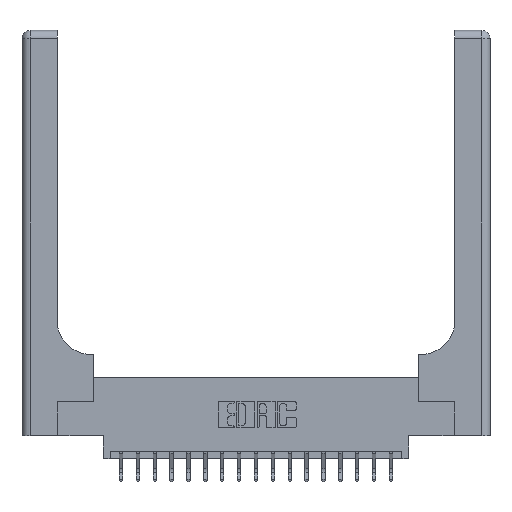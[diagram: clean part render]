
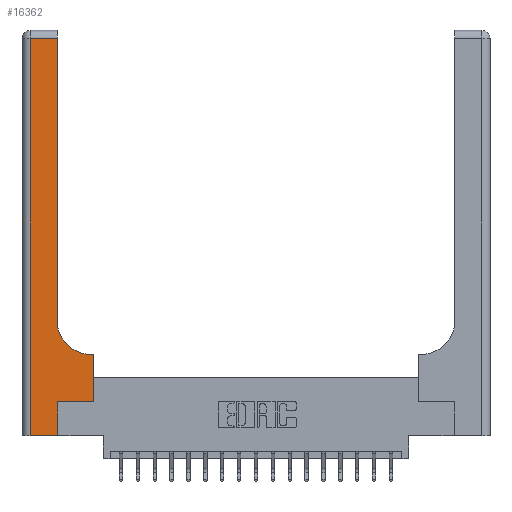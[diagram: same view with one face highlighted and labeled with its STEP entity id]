
A CAD part, top view. The second image highlights one B-rep face of the part: STEP entity #16362.
In plain terms, the highlighted planar face has unit normal (0, 0, 1).
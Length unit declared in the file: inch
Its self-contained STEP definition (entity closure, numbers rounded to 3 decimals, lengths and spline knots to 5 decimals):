
#475 = CARTESIAN_POINT ( 'NONE',  ( 0., 0., 0.37 ) ) ;
#522 = ORIENTED_EDGE ( 'NONE', *, *, #2065, .T. ) ;
#551 = DIRECTION ( 'NONE',  ( -1., 0., 0. ) ) ;
#961 = VERTEX_POINT ( 'NONE', #5490 ) ;
#1096 = DIRECTION ( 'NONE',  ( 0., 1., 0. ) ) ;
#1474 = DIRECTION ( 'NONE',  ( 0., 1., 0. ) ) ;
#1611 = VERTEX_POINT ( 'NONE', #2982 ) ;
#1693 = VECTOR ( 'NONE', #17607, 39.37008 ) ;
#1705 = VECTOR ( 'NONE', #16357, 39.37008 ) ;
#2053 = ORIENTED_EDGE ( 'NONE', *, *, #19436, .T. ) ;
#2065 = EDGE_CURVE ( 'NONE', #6285, #18009, #5100, .T. ) ;
#2177 = CARTESIAN_POINT ( 'NONE',  ( 0., 2.94, 0.37 ) ) ;
#2196 = CARTESIAN_POINT ( 'NONE',  ( 0.26, 0.6, 0.37 ) ) ;
#2361 = ORIENTED_EDGE ( 'NONE', *, *, #8511, .T. ) ;
#2476 = EDGE_CURVE ( 'NONE', #10745, #961, #14291, .T. ) ;
#2827 = CIRCLE ( 'NONE', #11440, 0.25 ) ;
#2853 = LINE ( 'NONE', #15486, #19802 ) ;
#2982 = CARTESIAN_POINT ( 'NONE',  ( 0.265, 0.25, 0.37 ) ) ;
#3101 = EDGE_CURVE ( 'NONE', #16613, #10745, #2853, .T. ) ;
#3130 = VERTEX_POINT ( 'NONE', #15181 ) ;
#3337 = CARTESIAN_POINT ( 'NONE',  ( 0.26, 0.85, 0.37 ) ) ;
#3581 = CARTESIAN_POINT ( 'NONE',  ( 0.26, 2.94, 0.37 ) ) ;
#4797 = CARTESIAN_POINT ( 'NONE',  ( 0.528, 0.6, 0.37 ) ) ;
#4808 = DIRECTION ( 'NONE',  ( 1., 0., 0. ) ) ;
#5100 = LINE ( 'NONE', #2196, #17167 ) ;
#5184 = VECTOR ( 'NONE', #4808, 39.37008 ) ;
#5490 = CARTESIAN_POINT ( 'NONE',  ( 0.06, 2.94, 0.37 ) ) ;
#5748 = EDGE_CURVE ( 'NONE', #961, #12472, #14971, .T. ) ;
#6152 = LINE ( 'NONE', #10940, #5184 ) ;
#6179 = DIRECTION ( 'NONE',  ( 0., 0., -1. ) ) ;
#6285 = VERTEX_POINT ( 'NONE', #4797 ) ;
#7074 = VERTEX_POINT ( 'NONE', #17645 ) ;
#8040 = DIRECTION ( 'NONE',  ( 1., 0., 0. ) ) ;
#8334 = FACE_OUTER_BOUND ( 'NONE', #10385, .T. ) ;
#8359 = CARTESIAN_POINT ( 'NONE',  ( 0.06, 3., 0.37 ) ) ;
#8511 = EDGE_CURVE ( 'NONE', #3130, #6285, #14005, .T. ) ;
#8544 = ORIENTED_EDGE ( 'NONE', *, *, #9188, .T. ) ;
#8663 = DIRECTION ( 'NONE',  ( 0., 0., -1. ) ) ;
#9188 = EDGE_CURVE ( 'NONE', #12472, #7074, #13227, .T. ) ;
#9408 = VECTOR ( 'NONE', #1474, 39.37008 ) ;
#10385 = EDGE_LOOP ( 'NONE', ( #17080, #19783, #10804, #8544, #2053, #17909, #2361, #522, #10898 ) ) ;
#10534 = EDGE_CURVE ( 'NONE', #18009, #16613, #2827, .T. ) ;
#10745 = VERTEX_POINT ( 'NONE', #3581 ) ;
#10804 = ORIENTED_EDGE ( 'NONE', *, *, #5748, .T. ) ;
#10898 = ORIENTED_EDGE ( 'NONE', *, *, #10534, .T. ) ;
#10940 = CARTESIAN_POINT ( 'NONE',  ( 0.265, 0.25, 0.37 ) ) ;
#11214 = LINE ( 'NONE', #14488, #1693 ) ;
#11440 = AXIS2_PLACEMENT_3D ( 'NONE', #15609, #6179, #8040 ) ;
#12072 = VECTOR ( 'NONE', #19526, 39.37008 ) ;
#12472 = VERTEX_POINT ( 'NONE', #16397 ) ;
#12721 = EDGE_CURVE ( 'NONE', #1611, #3130, #6152, .T. ) ;
#13227 = LINE ( 'NONE', #475, #12072 ) ;
#13960 = VECTOR ( 'NONE', #15074, 39.37008 ) ;
#14005 = LINE ( 'NONE', #18559, #9408 ) ;
#14291 = LINE ( 'NONE', #2177, #1705 ) ;
#14488 = CARTESIAN_POINT ( 'NONE',  ( 0.265, 0., 0.37 ) ) ;
#14971 = LINE ( 'NONE', #8359, #13960 ) ;
#15049 = CARTESIAN_POINT ( 'NONE',  ( 0., 3., 0.37 ) ) ;
#15074 = DIRECTION ( 'NONE',  ( 0., -1., 0. ) ) ;
#15181 = CARTESIAN_POINT ( 'NONE',  ( 0.528, 0.25, 0.37 ) ) ;
#15486 = CARTESIAN_POINT ( 'NONE',  ( 0.26, 3., 0.37 ) ) ;
#15609 = CARTESIAN_POINT ( 'NONE',  ( 0.51, 0.85, 0.37 ) ) ;
#15977 = DIRECTION ( 'NONE',  ( -1., 0., 0. ) ) ;
#16296 = PLANE ( 'NONE',  #17483 ) ;
#16357 = DIRECTION ( 'NONE',  ( -1., 0., 0. ) ) ;
#16362 = ADVANCED_FACE ( 'NONE', ( #8334 ), #16296, .F. ) ;
#16397 = CARTESIAN_POINT ( 'NONE',  ( 0.06, 0., 0.37 ) ) ;
#16613 = VERTEX_POINT ( 'NONE', #3337 ) ;
#17080 = ORIENTED_EDGE ( 'NONE', *, *, #3101, .T. ) ;
#17167 = VECTOR ( 'NONE', #15977, 39.37008 ) ;
#17483 = AXIS2_PLACEMENT_3D ( 'NONE', #15049, #8663, #551 ) ;
#17607 = DIRECTION ( 'NONE',  ( 0., 1., 0. ) ) ;
#17645 = CARTESIAN_POINT ( 'NONE',  ( 0.265, 0., 0.37 ) ) ;
#17909 = ORIENTED_EDGE ( 'NONE', *, *, #12721, .T. ) ;
#18009 = VERTEX_POINT ( 'NONE', #20189 ) ;
#18559 = CARTESIAN_POINT ( 'NONE',  ( 0.528, 0.25, 0.37 ) ) ;
#19436 = EDGE_CURVE ( 'NONE', #7074, #1611, #11214, .T. ) ;
#19526 = DIRECTION ( 'NONE',  ( 1., 0., 0. ) ) ;
#19783 = ORIENTED_EDGE ( 'NONE', *, *, #2476, .T. ) ;
#19802 = VECTOR ( 'NONE', #1096, 39.37008 ) ;
#20189 = CARTESIAN_POINT ( 'NONE',  ( 0.51, 0.6, 0.37 ) ) ;
